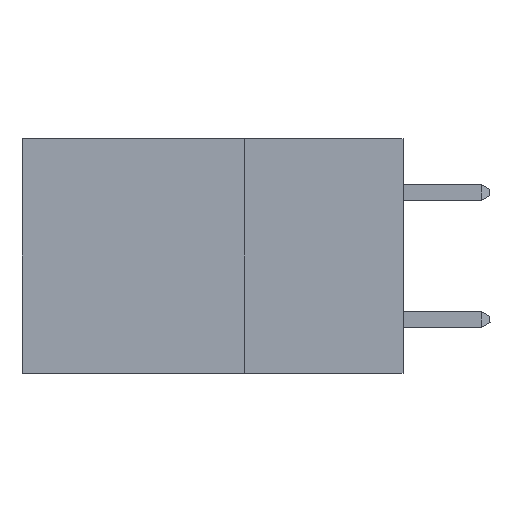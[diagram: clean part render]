
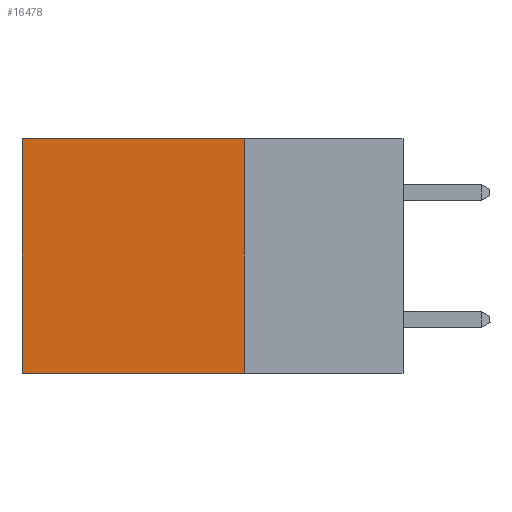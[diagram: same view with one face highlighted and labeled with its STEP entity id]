
A CAD part, left-side view. The second image highlights one B-rep face of the part: STEP entity #16478.
In plain terms, the highlighted planar face has unit normal (-1, 0, 0).
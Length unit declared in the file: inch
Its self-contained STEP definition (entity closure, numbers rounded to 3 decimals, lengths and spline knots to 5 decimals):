
#452 = CARTESIAN_POINT ( 'NONE',  ( 0.2875, 0.25, 0. ) ) ;
#1011 = ORIENTED_EDGE ( 'NONE', *, *, #7397, .F. ) ;
#1099 = DIRECTION ( 'NONE',  ( 0., 0., -1. ) ) ;
#1192 = LINE ( 'NONE', #14354, #18332 ) ;
#1430 = DIRECTION ( 'NONE',  ( 0., 1., 0. ) ) ;
#1999 = VECTOR ( 'NONE', #10311, 39.37008 ) ;
#2190 = EDGE_LOOP ( 'NONE', ( #5875, #1011, #8413, #18695 ) ) ;
#2862 = CARTESIAN_POINT ( 'NONE',  ( 0.2875, 0.25, 0. ) ) ;
#3751 = VERTEX_POINT ( 'NONE', #13264 ) ;
#5066 = EDGE_CURVE ( 'NONE', #12530, #19034, #1192, .T. ) ;
#5875 = ORIENTED_EDGE ( 'NONE', *, *, #8208, .T. ) ;
#5900 = CARTESIAN_POINT ( 'NONE',  ( 0.2875, 0.6, 0. ) ) ;
#7397 = EDGE_CURVE ( 'NONE', #19034, #3751, #10226, .T. ) ;
#7729 = AXIS2_PLACEMENT_3D ( 'NONE', #13772, #10463, #15306 ) ;
#7848 = FACE_OUTER_BOUND ( 'NONE', #2190, .T. ) ;
#8208 = EDGE_CURVE ( 'NONE', #13122, #3751, #13042, .T. ) ;
#8273 = EDGE_CURVE ( 'NONE', #12530, #13122, #13824, .T. ) ;
#8413 = ORIENTED_EDGE ( 'NONE', *, *, #5066, .F. ) ;
#9090 = VECTOR ( 'NONE', #1430, 39.37008 ) ;
#9315 = PLANE ( 'NONE',  #7729 ) ;
#9360 = DIRECTION ( 'NONE',  ( 0., 1., 0. ) ) ;
#10226 = LINE ( 'NONE', #11791, #9090 ) ;
#10311 = DIRECTION ( 'NONE',  ( 0., 0., -1. ) ) ;
#10463 = DIRECTION ( 'NONE',  ( 1., 0., 0. ) ) ;
#11791 = CARTESIAN_POINT ( 'NONE',  ( 0.2875, 0.25, -0.37 ) ) ;
#11923 = CARTESIAN_POINT ( 'NONE',  ( 0.2875, 0.6, 0. ) ) ;
#12530 = VERTEX_POINT ( 'NONE', #2862 ) ;
#13042 = LINE ( 'NONE', #11923, #1999 ) ;
#13122 = VERTEX_POINT ( 'NONE', #5900 ) ;
#13264 = CARTESIAN_POINT ( 'NONE',  ( 0.2875, 0.6, -0.37 ) ) ;
#13746 = VECTOR ( 'NONE', #9360, 39.37008 ) ;
#13772 = CARTESIAN_POINT ( 'NONE',  ( 0.2875, 0.25, 0. ) ) ;
#13824 = LINE ( 'NONE', #452, #13746 ) ;
#14354 = CARTESIAN_POINT ( 'NONE',  ( 0.2875, 0.25, 0. ) ) ;
#15306 = DIRECTION ( 'NONE',  ( 0., 0., -1. ) ) ;
#16385 = CARTESIAN_POINT ( 'NONE',  ( 0.2875, 0.25, -0.37 ) ) ;
#16478 = ADVANCED_FACE ( 'NONE', ( #7848 ), #9315, .F. ) ;
#18332 = VECTOR ( 'NONE', #1099, 39.37008 ) ;
#18695 = ORIENTED_EDGE ( 'NONE', *, *, #8273, .T. ) ;
#19034 = VERTEX_POINT ( 'NONE', #16385 ) ;
